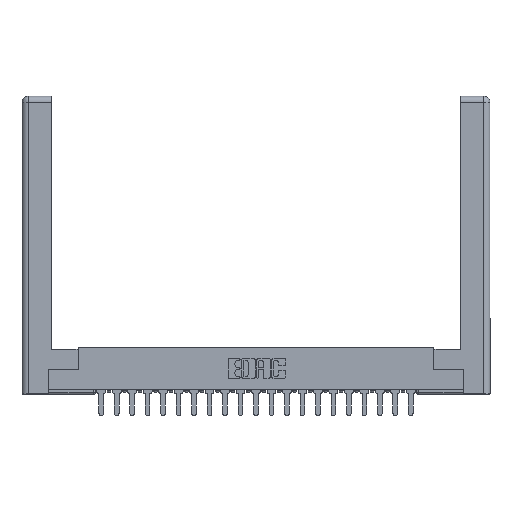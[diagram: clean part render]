
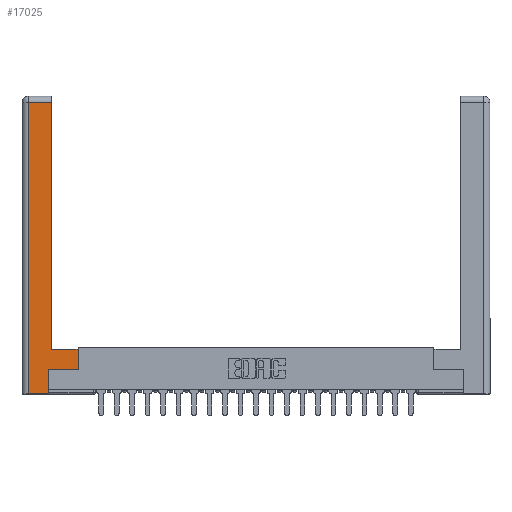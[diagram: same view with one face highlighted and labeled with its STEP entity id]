
A CAD part, top view. The second image highlights one B-rep face of the part: STEP entity #17025.
In plain terms, the highlighted planar face has unit normal (0, 0, 1).
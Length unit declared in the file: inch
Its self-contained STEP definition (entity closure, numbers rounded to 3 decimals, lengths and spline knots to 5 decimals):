
#56 = DIRECTION ( 'NONE',  ( -1., 0., 0. ) ) ;
#329 = DIRECTION ( 'NONE',  ( 0., 1., 0. ) ) ;
#400 = CARTESIAN_POINT ( 'NONE',  ( 0.295, 0.45, 0. ) ) ;
#630 = CARTESIAN_POINT ( 'NONE',  ( 0.565, 0.245, 0. ) ) ;
#761 = VERTEX_POINT ( 'NONE', #14111 ) ;
#1013 = VERTEX_POINT ( 'NONE', #11730 ) ;
#1519 = DIRECTION ( 'NONE',  ( -1., 0., 0. ) ) ;
#1735 = CARTESIAN_POINT ( 'NONE',  ( 0.295, 2.94, 0. ) ) ;
#1802 = DIRECTION ( 'NONE',  ( -1., 0., 0. ) ) ;
#2630 = ORIENTED_EDGE ( 'NONE', *, *, #7507, .T. ) ;
#2931 = CARTESIAN_POINT ( 'NONE',  ( 0.0615, 0., 0. ) ) ;
#3154 = CARTESIAN_POINT ( 'NONE',  ( 0., 0., 0. ) ) ;
#4013 = VERTEX_POINT ( 'NONE', #400 ) ;
#4325 = VECTOR ( 'NONE', #56, 39.37008 ) ;
#5379 = VERTEX_POINT ( 'NONE', #1735 ) ;
#5478 = CARTESIAN_POINT ( 'NONE',  ( 0.265, 0., 0. ) ) ;
#5753 = EDGE_CURVE ( 'NONE', #16226, #1013, #20074, .T. ) ;
#6134 = EDGE_CURVE ( 'NONE', #5379, #12665, #21181, .T. ) ;
#6509 = CARTESIAN_POINT ( 'NONE',  ( 0.0615, 2.94, 0. ) ) ;
#6751 = VECTOR ( 'NONE', #17434, 39.37008 ) ;
#6962 = VECTOR ( 'NONE', #1802, 39.37008 ) ;
#7231 = ORIENTED_EDGE ( 'NONE', *, *, #16364, .T. ) ;
#7507 = EDGE_CURVE ( 'NONE', #4013, #5379, #21110, .T. ) ;
#7939 = ORIENTED_EDGE ( 'NONE', *, *, #22576, .T. ) ;
#8327 = ORIENTED_EDGE ( 'NONE', *, *, #12637, .T. ) ;
#8436 = CARTESIAN_POINT ( 'NONE',  ( 0.295, 3., 0. ) ) ;
#8713 = LINE ( 'NONE', #17515, #6751 ) ;
#8878 = EDGE_LOOP ( 'NONE', ( #2630, #17064, #7939, #8327, #20936, #7231, #16673, #23019 ) ) ;
#9225 = CARTESIAN_POINT ( 'NONE',  ( 0.565, 0.45, 0. ) ) ;
#10062 = VECTOR ( 'NONE', #18667, 39.37008 ) ;
#11730 = CARTESIAN_POINT ( 'NONE',  ( 0.565, 0.45, 0. ) ) ;
#11933 = VECTOR ( 'NONE', #329, 39.37008 ) ;
#12637 = EDGE_CURVE ( 'NONE', #21098, #761, #22895, .T. ) ;
#12665 = VERTEX_POINT ( 'NONE', #19841 ) ;
#13941 = VERTEX_POINT ( 'NONE', #15771 ) ;
#14111 = CARTESIAN_POINT ( 'NONE',  ( 0.265, 0., 0. ) ) ;
#14551 = CARTESIAN_POINT ( 'NONE',  ( 0.0615, 0., 0. ) ) ;
#15557 = AXIS2_PLACEMENT_3D ( 'NONE', #3154, #17486, #1519 ) ;
#15771 = CARTESIAN_POINT ( 'NONE',  ( 0.265, 0.245, 0. ) ) ;
#16174 = DIRECTION ( 'NONE',  ( 1., 0., 0. ) ) ;
#16226 = VERTEX_POINT ( 'NONE', #630 ) ;
#16364 = EDGE_CURVE ( 'NONE', #13941, #16226, #8713, .T. ) ;
#16673 = ORIENTED_EDGE ( 'NONE', *, *, #5753, .T. ) ;
#17025 = ADVANCED_FACE ( 'NONE', ( #18518 ), #21267, .F. ) ;
#17064 = ORIENTED_EDGE ( 'NONE', *, *, #6134, .T. ) ;
#17394 = EDGE_CURVE ( 'NONE', #761, #13941, #19050, .T. ) ;
#17434 = DIRECTION ( 'NONE',  ( 1., 0., 0. ) ) ;
#17486 = DIRECTION ( 'NONE',  ( 0., 0., -1. ) ) ;
#17515 = CARTESIAN_POINT ( 'NONE',  ( 0.565, 0.245, 0. ) ) ;
#18518 = FACE_OUTER_BOUND ( 'NONE', #8878, .T. ) ;
#18667 = DIRECTION ( 'NONE',  ( 0., 1., 0. ) ) ;
#19050 = LINE ( 'NONE', #22335, #10062 ) ;
#19841 = CARTESIAN_POINT ( 'NONE',  ( 0.0615, 2.94, 0. ) ) ;
#20074 = LINE ( 'NONE', #9225, #11933 ) ;
#20378 = LINE ( 'NONE', #2931, #23166 ) ;
#20639 = DIRECTION ( 'NONE',  ( 0., -1., 0. ) ) ;
#20922 = EDGE_CURVE ( 'NONE', #1013, #4013, #21855, .T. ) ;
#20936 = ORIENTED_EDGE ( 'NONE', *, *, #17394, .T. ) ;
#20991 = DIRECTION ( 'NONE',  ( 0., 1., 0. ) ) ;
#21098 = VERTEX_POINT ( 'NONE', #14551 ) ;
#21110 = LINE ( 'NONE', #8436, #23051 ) ;
#21181 = LINE ( 'NONE', #6509, #4325 ) ;
#21216 = VECTOR ( 'NONE', #16174, 39.37008 ) ;
#21267 = PLANE ( 'NONE',  #15557 ) ;
#21381 = CARTESIAN_POINT ( 'NONE',  ( 0.295, 0.45, 0. ) ) ;
#21855 = LINE ( 'NONE', #21381, #6962 ) ;
#22335 = CARTESIAN_POINT ( 'NONE',  ( 0.265, 0.245, 0. ) ) ;
#22576 = EDGE_CURVE ( 'NONE', #12665, #21098, #20378, .T. ) ;
#22895 = LINE ( 'NONE', #5478, #21216 ) ;
#23019 = ORIENTED_EDGE ( 'NONE', *, *, #20922, .T. ) ;
#23051 = VECTOR ( 'NONE', #20991, 39.37008 ) ;
#23166 = VECTOR ( 'NONE', #20639, 39.37008 ) ;
